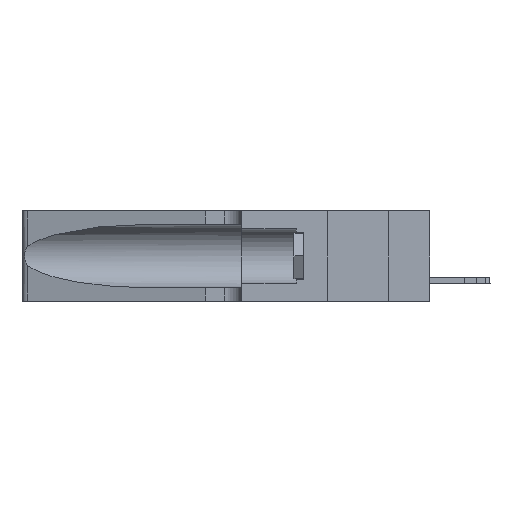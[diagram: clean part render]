
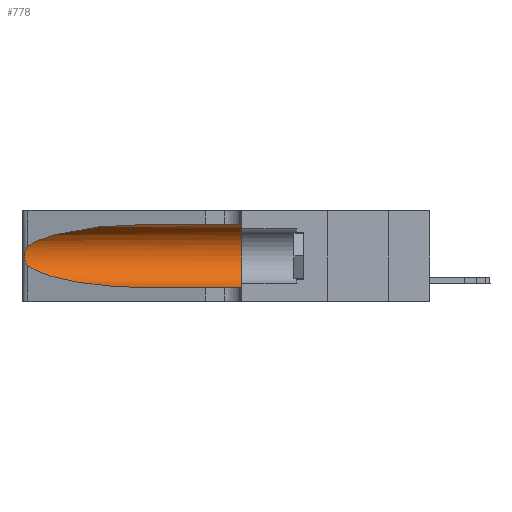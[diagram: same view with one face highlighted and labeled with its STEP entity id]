
A CAD part, left-side view. The second image highlights one B-rep face of the part: STEP entity #778.
In plain terms, the highlighted cylindrical face has radius 3.308 mm (diameter 6.617 mm), a partial arc.
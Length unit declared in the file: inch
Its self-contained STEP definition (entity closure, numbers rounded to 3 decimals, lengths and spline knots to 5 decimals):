
#778 = ADVANCED_FACE ( 'NONE', ( #1821 ), #20483, .F. ) ;
#1098 =( BOUNDED_CURVE ( )  B_SPLINE_CURVE ( 3, ( #13558, #33186, #13681, #5016 ),
 .UNSPECIFIED., .F., .F. ) 
 B_SPLINE_CURVE_WITH_KNOTS ( ( 4, 4 ),
 ( 3.44316, 4.71239 ),
 .UNSPECIFIED. ) 
 CURVE ( )  GEOMETRIC_REPRESENTATION_ITEM ( )  RATIONAL_B_SPLINE_CURVE ( ( 1., 0.87, 0.87, 1. ) ) 
 REPRESENTATION_ITEM ( '' )  );
#1218 = ORIENTED_EDGE ( 'NONE', *, *, #27543, .F. ) ;
#1821 = FACE_OUTER_BOUND ( 'NONE', #10884, .T. ) ;
#2232 = CARTESIAN_POINT ( 'NONE',  ( 0.1305, 0.35, 0.31525 ) ) ;
#3171 = CARTESIAN_POINT ( 'NONE',  ( 0.2373, 1.15595, 0.28018 ) ) ;
#4002 = EDGE_CURVE ( 'NONE', #34061, #21339, #1098, .T. ) ;
#5016 = CARTESIAN_POINT ( 'NONE',  ( 0.1305, 0.72297, 0.05475 ) ) ;
#5312 = CARTESIAN_POINT ( 'NONE',  ( 0.1305, 0.72297, 0.31525 ) ) ;
#6308 = CARTESIAN_POINT ( 'NONE',  ( 0.25787, 1.23484, 0.2124 ) ) ;
#6949 = ORIENTED_EDGE ( 'NONE', *, *, #22574, .F. ) ;
#7384 = CARTESIAN_POINT ( 'NONE',  ( 0.1305, 0.35, 0.05475 ) ) ;
#7683 = CARTESIAN_POINT ( 'NONE',  ( 0.1305, 0.72297, 0.31525 ) ) ;
#7692 = CARTESIAN_POINT ( 'NONE',  ( 0.25487, 1.22718, 0.22369 ) ) ;
#8066 = VERTEX_POINT ( 'NONE', #7384 ) ;
#8126 = DIRECTION ( 'NONE',  ( 0., -1., 0. ) ) ;
#8271 = CARTESIAN_POINT ( 'NONE',  ( 0.25854, 1.2359, 0.20912 ) ) ;
#8276 = VERTEX_POINT ( 'NONE', #7683 ) ;
#8578 = VECTOR ( 'NONE', #28093, 39.37008 ) ;
#9006 = CARTESIAN_POINT ( 'NONE',  ( 0.25487, 1.22718, 0.14631 ) ) ;
#10249 = DIRECTION ( 'NONE',  ( 0., 1., 0. ) ) ;
#10483 = CARTESIAN_POINT ( 'NONE',  ( 0.26075, 1.23896, 0.178 ) ) ;
#10609 = CARTESIAN_POINT ( 'NONE',  ( 0.25789, 1.23486, 0.15765 ) ) ;
#10627 = DIRECTION ( 'NONE',  ( 0., 0., -1. ) ) ;
#10842 = VERTEX_POINT ( 'NONE', #7692 ) ;
#10884 = EDGE_LOOP ( 'NONE', ( #15303, #17546, #17112, #25636, #6949, #1218 ) ) ;
#11419 = CARTESIAN_POINT ( 'NONE',  ( 0.25487, 1.22718, 0.22369 ) ) ;
#12938 = EDGE_CURVE ( 'NONE', #21339, #8066, #30060, .T. ) ;
#13379 = CIRCLE ( 'NONE', #15476, 0.13025 ) ;
#13558 = CARTESIAN_POINT ( 'NONE',  ( 0.25487, 1.22718, 0.14631 ) ) ;
#13681 = CARTESIAN_POINT ( 'NONE',  ( 0.18966, 0.96281, 0.05475 ) ) ;
#13748 = CARTESIAN_POINT ( 'NONE',  ( 0.1305, 1.61858, 0.185 ) ) ;
#13777 = LINE ( 'NONE', #26652, #24959 ) ;
#14099 = CARTESIAN_POINT ( 'NONE',  ( 0.18966, 0.96281, 0.31525 ) ) ;
#15303 = ORIENTED_EDGE ( 'NONE', *, *, #21494, .T. ) ;
#15476 = AXIS2_PLACEMENT_3D ( 'NONE', #21229, #10249, #36329 ) ;
#15493 = VERTEX_POINT ( 'NONE', #2232 ) ;
#17041 = CARTESIAN_POINT ( 'NONE',  ( 0.25639, 1.23186, 0.15144 ) ) ;
#17112 = ORIENTED_EDGE ( 'NONE', *, *, #4002, .T. ) ;
#17546 = ORIENTED_EDGE ( 'NONE', *, *, #34412, .T. ) ;
#19582 = CARTESIAN_POINT ( 'NONE',  ( 0.25555, 1.22994, 0.2215 ) ) ;
#20483 = CYLINDRICAL_SURFACE ( 'NONE', #24229, 0.13025 ) ;
#21229 = CARTESIAN_POINT ( 'NONE',  ( 0.1305, 0.35, 0.185 ) ) ;
#21339 = VERTEX_POINT ( 'NONE', #23429 ) ;
#21494 = EDGE_CURVE ( 'NONE', #8276, #10842, #31917, .T. ) ;
#21864 = CARTESIAN_POINT ( 'NONE',  ( 0.26075, 1.23896, 0.19203 ) ) ;
#22574 = EDGE_CURVE ( 'NONE', #15493, #8066, #13379, .T. ) ;
#23429 = CARTESIAN_POINT ( 'NONE',  ( 0.1305, 0.72297, 0.05475 ) ) ;
#23901 = DIRECTION ( 'NONE',  ( 0., -1., 0. ) ) ;
#24229 = AXIS2_PLACEMENT_3D ( 'NONE', #13748, #8126, #10627 ) ;
#24464 = CARTESIAN_POINT ( 'NONE',  ( 0.25487, 1.22718, 0.22369 ) ) ;
#24882 = CARTESIAN_POINT ( 'NONE',  ( 0.25856, 1.23593, 0.16098 ) ) ;
#24959 = VECTOR ( 'NONE', #23901, 39.37008 ) ;
#25378 = CARTESIAN_POINT ( 'NONE',  ( 0.25487, 1.22718, 0.14631 ) ) ;
#25636 = ORIENTED_EDGE ( 'NONE', *, *, #12938, .T. ) ;
#26652 = CARTESIAN_POINT ( 'NONE',  ( 0.1305, 1.61858, 0.31525 ) ) ;
#27543 = EDGE_CURVE ( 'NONE', #8276, #15493, #13777, .T. ) ;
#27624 = B_SPLINE_CURVE_WITH_KNOTS ( 'NONE', 3,
 ( #24464, #19582, #33459, #6308, #8271, #33358, #21864, #10483, #30485, #24882, #10609, #17041, #31095, #25378 ),
 .UNSPECIFIED., .F., .F.,
 ( 4, 2, 2, 2, 2, 2, 4 ),
 ( 0., 0.00027, 0.00053, 0.00107, 0.0016, 0.00187, 0.00214 ),
 .UNSPECIFIED. ) ;
#28093 = DIRECTION ( 'NONE',  ( 0., -1., 0. ) ) ;
#30060 = LINE ( 'NONE', #33701, #8578 ) ;
#30485 = CARTESIAN_POINT ( 'NONE',  ( 0.26017, 1.23833, 0.17102 ) ) ;
#31095 = CARTESIAN_POINT ( 'NONE',  ( 0.25555, 1.22993, 0.14849 ) ) ;
#31917 =( BOUNDED_CURVE ( )  B_SPLINE_CURVE ( 3, ( #5312, #14099, #3171, #11419 ),
 .UNSPECIFIED., .F., .F. ) 
 B_SPLINE_CURVE_WITH_KNOTS ( ( 4, 4 ),
 ( 1.5708, 2.84003 ),
 .UNSPECIFIED. ) 
 CURVE ( )  GEOMETRIC_REPRESENTATION_ITEM ( )  RATIONAL_B_SPLINE_CURVE ( ( 1., 0.87, 0.87, 1. ) ) 
 REPRESENTATION_ITEM ( '' )  );
#33186 = CARTESIAN_POINT ( 'NONE',  ( 0.2373, 1.15595, 0.08982 ) ) ;
#33358 = CARTESIAN_POINT ( 'NONE',  ( 0.26018, 1.23835, 0.19895 ) ) ;
#33459 = CARTESIAN_POINT ( 'NONE',  ( 0.25639, 1.23184, 0.21858 ) ) ;
#33701 = CARTESIAN_POINT ( 'NONE',  ( 0.1305, 1.61858, 0.05475 ) ) ;
#34061 = VERTEX_POINT ( 'NONE', #9006 ) ;
#34412 = EDGE_CURVE ( 'NONE', #10842, #34061, #27624, .T. ) ;
#36329 = DIRECTION ( 'NONE',  ( 0., 0., 1. ) ) ;
